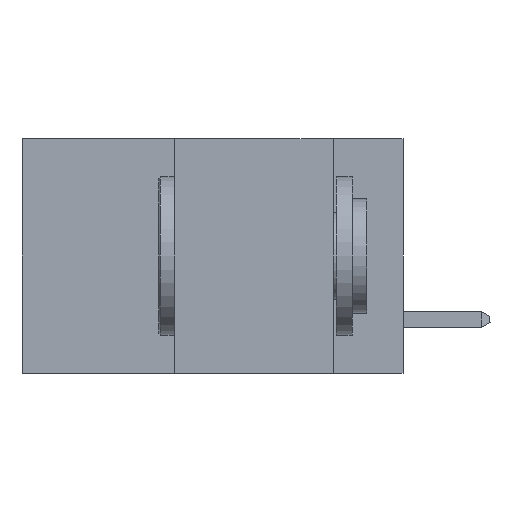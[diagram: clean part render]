
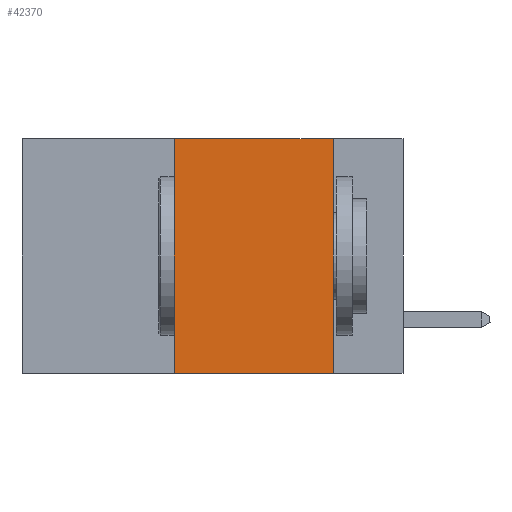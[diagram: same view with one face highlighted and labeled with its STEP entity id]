
A CAD part, left-side view. The second image highlights one B-rep face of the part: STEP entity #42370.
In plain terms, the highlighted planar face has unit normal (-1, 0, 0).
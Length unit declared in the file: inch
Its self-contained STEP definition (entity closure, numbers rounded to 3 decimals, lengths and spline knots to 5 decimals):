
#1039 = DIRECTION ( 'NONE',  ( 0., 0., -1. ) ) ;
#1261 = CARTESIAN_POINT ( 'NONE',  ( 0., 0.36, 0. ) ) ;
#2281 = DIRECTION ( 'NONE',  ( 0., 0., -1. ) ) ;
#5321 = DIRECTION ( 'NONE',  ( 0., -1., 0. ) ) ;
#5409 = VECTOR ( 'NONE', #1039, 39.37008 ) ;
#5829 = PLANE ( 'NONE',  #37469 ) ;
#8022 = EDGE_LOOP ( 'NONE', ( #43957, #29340, #44166, #14690 ) ) ;
#8649 = VECTOR ( 'NONE', #5321, 39.37008 ) ;
#8881 = VERTEX_POINT ( 'NONE', #1261 ) ;
#9789 = CARTESIAN_POINT ( 'NONE',  ( 0., 0.36, 0. ) ) ;
#12058 = CARTESIAN_POINT ( 'NONE',  ( 0., 0.6, -0.37 ) ) ;
#14690 = ORIENTED_EDGE ( 'NONE', *, *, #29518, .T. ) ;
#16275 = LINE ( 'NONE', #12058, #8649 ) ;
#17614 = VERTEX_POINT ( 'NONE', #28625 ) ;
#21623 = DIRECTION ( 'NONE',  ( 0., -1., 0. ) ) ;
#21925 = VERTEX_POINT ( 'NONE', #25241 ) ;
#22297 = EDGE_CURVE ( 'NONE', #8881, #26636, #39306, .T. ) ;
#22374 = LINE ( 'NONE', #25667, #5409 ) ;
#25241 = CARTESIAN_POINT ( 'NONE',  ( 0., 0.36, -0.37 ) ) ;
#25667 = CARTESIAN_POINT ( 'NONE',  ( 0., 0.11, 0. ) ) ;
#26636 = VERTEX_POINT ( 'NONE', #43575 ) ;
#28625 = CARTESIAN_POINT ( 'NONE',  ( 0., 0.11, -0.37 ) ) ;
#29340 = ORIENTED_EDGE ( 'NONE', *, *, #22297, .F. ) ;
#29518 = EDGE_CURVE ( 'NONE', #21925, #17614, #16275, .T. ) ;
#30172 = EDGE_CURVE ( 'NONE', #21925, #8881, #37143, .T. ) ;
#34143 = FACE_OUTER_BOUND ( 'NONE', #8022, .T. ) ;
#36937 = DIRECTION ( 'NONE',  ( 1., 0., 0. ) ) ;
#37143 = LINE ( 'NONE', #9789, #41532 ) ;
#37469 = AXIS2_PLACEMENT_3D ( 'NONE', #40613, #36937, #2281 ) ;
#37506 = DIRECTION ( 'NONE',  ( 0., 0., 1. ) ) ;
#38276 = VECTOR ( 'NONE', #21623, 39.37008 ) ;
#39280 = EDGE_CURVE ( 'NONE', #26636, #17614, #22374, .T. ) ;
#39306 = LINE ( 'NONE', #40532, #38276 ) ;
#40532 = CARTESIAN_POINT ( 'NONE',  ( 0., 0.6, 0. ) ) ;
#40613 = CARTESIAN_POINT ( 'NONE',  ( 0., 0.6, 0. ) ) ;
#41532 = VECTOR ( 'NONE', #37506, 39.37008 ) ;
#42370 = ADVANCED_FACE ( 'NONE', ( #34143 ), #5829, .F. ) ;
#43575 = CARTESIAN_POINT ( 'NONE',  ( 0., 0.11, 0. ) ) ;
#43957 = ORIENTED_EDGE ( 'NONE', *, *, #39280, .F. ) ;
#44166 = ORIENTED_EDGE ( 'NONE', *, *, #30172, .F. ) ;
